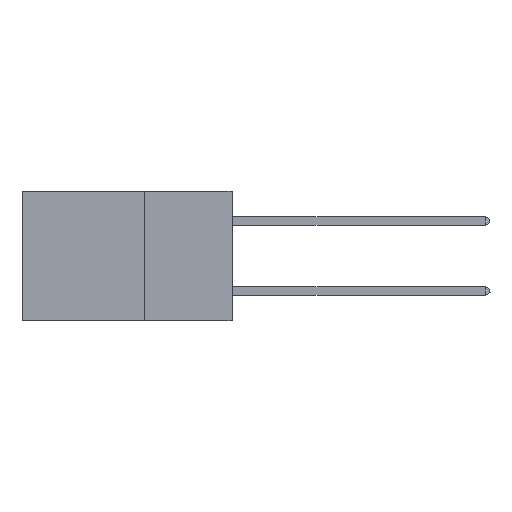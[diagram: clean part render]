
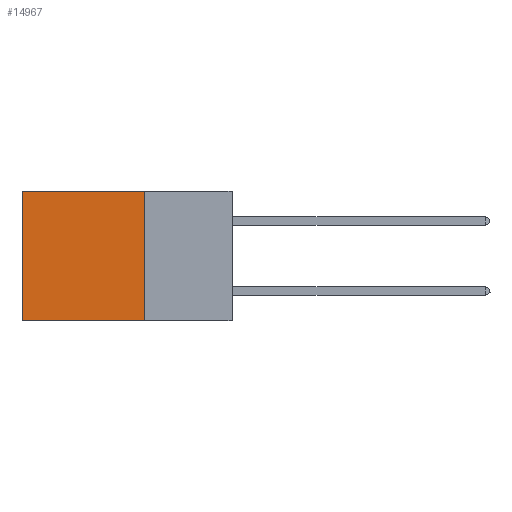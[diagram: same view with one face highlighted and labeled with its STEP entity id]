
A CAD part, left-side view. The second image highlights one B-rep face of the part: STEP entity #14967.
In plain terms, the highlighted planar face has unit normal (-1, 0, 0).
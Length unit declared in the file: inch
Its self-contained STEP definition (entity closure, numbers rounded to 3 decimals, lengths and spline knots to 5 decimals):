
#178 = VECTOR ( 'NONE', #10415, 39.37008 ) ;
#1456 = ORIENTED_EDGE ( 'NONE', *, *, #19832, .F. ) ;
#1609 = VECTOR ( 'NONE', #19268, 39.37008 ) ;
#3093 = ORIENTED_EDGE ( 'NONE', *, *, #4187, .T. ) ;
#4187 = EDGE_CURVE ( 'NONE', #14089, #21065, #7249, .T. ) ;
#4192 = EDGE_LOOP ( 'NONE', ( #12763, #14608, #1456, #3093 ) ) ;
#5212 = CARTESIAN_POINT ( 'NONE',  ( 0.2875, 0.25, 0. ) ) ;
#5768 = EDGE_CURVE ( 'NONE', #14698, #6783, #12088, .T. ) ;
#6431 = CARTESIAN_POINT ( 'NONE',  ( 0.2875, 0.25, 0. ) ) ;
#6783 = VERTEX_POINT ( 'NONE', #8693 ) ;
#7249 = LINE ( 'NONE', #5212, #7764 ) ;
#7439 = DIRECTION ( 'NONE',  ( 1., 0., 0. ) ) ;
#7703 = VECTOR ( 'NONE', #10670, 39.37008 ) ;
#7764 = VECTOR ( 'NONE', #14912, 39.37008 ) ;
#8204 = CARTESIAN_POINT ( 'NONE',  ( 0.2875, 0.25, -0.37 ) ) ;
#8693 = CARTESIAN_POINT ( 'NONE',  ( 0.2875, 0.6, -0.37 ) ) ;
#8791 = CARTESIAN_POINT ( 'NONE',  ( 0.2875, 0.25, -0.37 ) ) ;
#9482 = LINE ( 'NONE', #20275, #178 ) ;
#9846 = LINE ( 'NONE', #18996, #1609 ) ;
#10415 = DIRECTION ( 'NONE',  ( 0., 0., -1. ) ) ;
#10670 = DIRECTION ( 'NONE',  ( 0., 1., 0. ) ) ;
#12088 = LINE ( 'NONE', #8791, #7703 ) ;
#12763 = ORIENTED_EDGE ( 'NONE', *, *, #16341, .T. ) ;
#12769 = AXIS2_PLACEMENT_3D ( 'NONE', #17402, #7439, #13991 ) ;
#13991 = DIRECTION ( 'NONE',  ( 0., 0., -1. ) ) ;
#14089 = VERTEX_POINT ( 'NONE', #6431 ) ;
#14426 = FACE_OUTER_BOUND ( 'NONE', #4192, .T. ) ;
#14608 = ORIENTED_EDGE ( 'NONE', *, *, #5768, .F. ) ;
#14698 = VERTEX_POINT ( 'NONE', #8204 ) ;
#14912 = DIRECTION ( 'NONE',  ( 0., 1., 0. ) ) ;
#14967 = ADVANCED_FACE ( 'NONE', ( #14426 ), #18910, .F. ) ;
#16341 = EDGE_CURVE ( 'NONE', #21065, #6783, #9482, .T. ) ;
#17402 = CARTESIAN_POINT ( 'NONE',  ( 0.2875, 0.25, 0. ) ) ;
#18910 = PLANE ( 'NONE',  #12769 ) ;
#18996 = CARTESIAN_POINT ( 'NONE',  ( 0.2875, 0.25, 0. ) ) ;
#19268 = DIRECTION ( 'NONE',  ( 0., 0., -1. ) ) ;
#19832 = EDGE_CURVE ( 'NONE', #14089, #14698, #9846, .T. ) ;
#20275 = CARTESIAN_POINT ( 'NONE',  ( 0.2875, 0.6, 0. ) ) ;
#20996 = CARTESIAN_POINT ( 'NONE',  ( 0.2875, 0.6, 0. ) ) ;
#21065 = VERTEX_POINT ( 'NONE', #20996 ) ;
